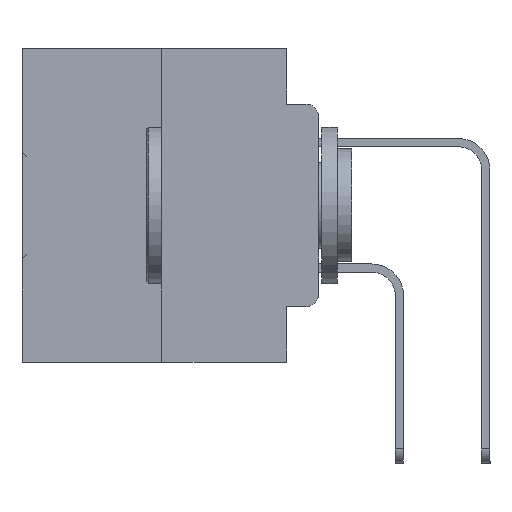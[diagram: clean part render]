
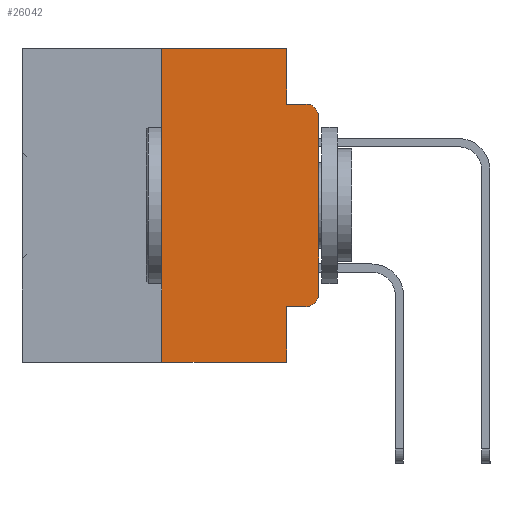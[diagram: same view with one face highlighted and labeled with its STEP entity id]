
A CAD part, left-side view. The second image highlights one B-rep face of the part: STEP entity #26042.
In plain terms, the highlighted planar face has unit normal (-1, 0, 0).
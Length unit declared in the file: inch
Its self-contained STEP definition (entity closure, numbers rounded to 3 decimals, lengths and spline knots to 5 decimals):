
#240 = CARTESIAN_POINT ( 'NONE',  ( 0., 0., 0. ) ) ;
#330 = VECTOR ( 'NONE', #24345, 39.37008 ) ;
#2341 = LINE ( 'NONE', #14823, #23618 ) ;
#2370 = ORIENTED_EDGE ( 'NONE', *, *, #24850, .F. ) ;
#2876 = DIRECTION ( 'NONE',  ( 0., 0., 1. ) ) ;
#2922 = CARTESIAN_POINT ( 'NONE',  ( 0., 0.051, -0.5 ) ) ;
#3687 = CIRCLE ( 'NONE', #19237, 0.02 ) ;
#4268 = CARTESIAN_POINT ( 'NONE',  ( 0., 0., -0.3915 ) ) ;
#4388 = LINE ( 'NONE', #28721, #18410 ) ;
#5376 = CARTESIAN_POINT ( 'NONE',  ( 0., 0.02, -0.4115 ) ) ;
#6795 = ORIENTED_EDGE ( 'NONE', *, *, #19258, .T. ) ;
#7227 = VERTEX_POINT ( 'NONE', #17693 ) ;
#7943 = VERTEX_POINT ( 'NONE', #12831 ) ;
#8115 = VERTEX_POINT ( 'NONE', #35006 ) ;
#8213 = VERTEX_POINT ( 'NONE', #5376 ) ;
#8551 = CARTESIAN_POINT ( 'NONE',  ( 0., 0.02, -0.1085 ) ) ;
#8991 = ORIENTED_EDGE ( 'NONE', *, *, #18989, .F. ) ;
#9557 = VECTOR ( 'NONE', #20720, 39.37008 ) ;
#9580 = CARTESIAN_POINT ( 'NONE',  ( 0., 0.25, 0. ) ) ;
#9655 = VECTOR ( 'NONE', #21869, 39.37008 ) ;
#9898 = AXIS2_PLACEMENT_3D ( 'NONE', #19679, #14055, #25079 ) ;
#10693 = CARTESIAN_POINT ( 'NONE',  ( 0., 0.473, 0. ) ) ;
#11161 = VERTEX_POINT ( 'NONE', #4268 ) ;
#11402 = DIRECTION ( 'NONE',  ( 0., 0., -1. ) ) ;
#12434 = FACE_OUTER_BOUND ( 'NONE', #19178, .T. ) ;
#12489 = DIRECTION ( 'NONE',  ( -1., 0., 0. ) ) ;
#12831 = CARTESIAN_POINT ( 'NONE',  ( 0., 0.02, -0.0885 ) ) ;
#13677 = EDGE_CURVE ( 'NONE', #7227, #7943, #16080, .T. ) ;
#14055 = DIRECTION ( 'NONE',  ( 1., 0., 0. ) ) ;
#14742 = ORIENTED_EDGE ( 'NONE', *, *, #16706, .F. ) ;
#14823 = CARTESIAN_POINT ( 'NONE',  ( 0., 0.25, 0. ) ) ;
#15649 = DIRECTION ( 'NONE',  ( 0., -1., 0. ) ) ;
#15818 = VECTOR ( 'NONE', #33776, 39.37008 ) ;
#16080 = CIRCLE ( 'NONE', #21864, 0.02 ) ;
#16270 = LINE ( 'NONE', #10693, #330 ) ;
#16706 = EDGE_CURVE ( 'NONE', #30278, #7943, #29245, .T. ) ;
#16755 = EDGE_CURVE ( 'NONE', #8213, #11161, #3687, .T. ) ;
#17120 = LINE ( 'NONE', #32486, #9655 ) ;
#17693 = CARTESIAN_POINT ( 'NONE',  ( 0., 0., -0.1085 ) ) ;
#18007 = CARTESIAN_POINT ( 'NONE',  ( 0., 0.051, 0. ) ) ;
#18277 = LINE ( 'NONE', #240, #24588 ) ;
#18410 = VECTOR ( 'NONE', #31454, 39.37008 ) ;
#18660 = LINE ( 'NONE', #29017, #32910 ) ;
#18989 = EDGE_CURVE ( 'NONE', #23869, #30278, #4388, .T. ) ;
#19041 = ORIENTED_EDGE ( 'NONE', *, *, #32118, .T. ) ;
#19178 = EDGE_LOOP ( 'NONE', ( #21129, #35382, #14742, #8991, #30756, #2370, #19041, #27809, #6795, #29479 ) ) ;
#19237 = AXIS2_PLACEMENT_3D ( 'NONE', #28678, #12489, #31419 ) ;
#19258 = EDGE_CURVE ( 'NONE', #32862, #8213, #17120, .T. ) ;
#19679 = CARTESIAN_POINT ( 'NONE',  ( 0., 0.473, 0. ) ) ;
#20578 = EDGE_CURVE ( 'NONE', #32862, #24183, #31293, .T. ) ;
#20720 = DIRECTION ( 'NONE',  ( 0., 0., -1. ) ) ;
#21129 = ORIENTED_EDGE ( 'NONE', *, *, #31504, .T. ) ;
#21864 = AXIS2_PLACEMENT_3D ( 'NONE', #8551, #27673, #11402 ) ;
#21869 = DIRECTION ( 'NONE',  ( 0., -1., 0. ) ) ;
#22399 = PLANE ( 'NONE',  #9898 ) ;
#22901 = CARTESIAN_POINT ( 'NONE',  ( 0., 0.051, -0.0885 ) ) ;
#23618 = VECTOR ( 'NONE', #2876, 39.37008 ) ;
#23869 = VERTEX_POINT ( 'NONE', #31746 ) ;
#24183 = VERTEX_POINT ( 'NONE', #2922 ) ;
#24345 = DIRECTION ( 'NONE',  ( 0., -1., 0. ) ) ;
#24588 = VECTOR ( 'NONE', #25276, 39.37008 ) ;
#24850 = EDGE_CURVE ( 'NONE', #8115, #26281, #2341, .T. ) ;
#25079 = DIRECTION ( 'NONE',  ( 0., 0., -1. ) ) ;
#25276 = DIRECTION ( 'NONE',  ( 0., 0., 1. ) ) ;
#25693 = CARTESIAN_POINT ( 'NONE',  ( 0., 0.051, -0.0885 ) ) ;
#26042 = ADVANCED_FACE ( 'NONE', ( #12434 ), #22399, .F. ) ;
#26281 = VERTEX_POINT ( 'NONE', #9580 ) ;
#27673 = DIRECTION ( 'NONE',  ( -1., 0., 0. ) ) ;
#27809 = ORIENTED_EDGE ( 'NONE', *, *, #20578, .F. ) ;
#28678 = CARTESIAN_POINT ( 'NONE',  ( 0., 0.02, -0.3915 ) ) ;
#28721 = CARTESIAN_POINT ( 'NONE',  ( 0., 0.051, 0. ) ) ;
#29017 = CARTESIAN_POINT ( 'NONE',  ( 0., 0.473, -0.5 ) ) ;
#29245 = LINE ( 'NONE', #25693, #15818 ) ;
#29326 = EDGE_CURVE ( 'NONE', #26281, #23869, #16270, .T. ) ;
#29479 = ORIENTED_EDGE ( 'NONE', *, *, #16755, .T. ) ;
#30278 = VERTEX_POINT ( 'NONE', #22901 ) ;
#30756 = ORIENTED_EDGE ( 'NONE', *, *, #29326, .F. ) ;
#31293 = LINE ( 'NONE', #18007, #9557 ) ;
#31419 = DIRECTION ( 'NONE',  ( 0., 0., -1. ) ) ;
#31454 = DIRECTION ( 'NONE',  ( 0., 0., -1. ) ) ;
#31504 = EDGE_CURVE ( 'NONE', #11161, #7227, #18277, .T. ) ;
#31746 = CARTESIAN_POINT ( 'NONE',  ( 0., 0.051, 0. ) ) ;
#32118 = EDGE_CURVE ( 'NONE', #8115, #24183, #18660, .T. ) ;
#32486 = CARTESIAN_POINT ( 'NONE',  ( 0., 0.051, -0.4115 ) ) ;
#32862 = VERTEX_POINT ( 'NONE', #34630 ) ;
#32910 = VECTOR ( 'NONE', #15649, 39.37008 ) ;
#33776 = DIRECTION ( 'NONE',  ( 0., -1., 0. ) ) ;
#34630 = CARTESIAN_POINT ( 'NONE',  ( 0., 0.051, -0.4115 ) ) ;
#35006 = CARTESIAN_POINT ( 'NONE',  ( 0., 0.25, -0.5 ) ) ;
#35382 = ORIENTED_EDGE ( 'NONE', *, *, #13677, .T. ) ;
